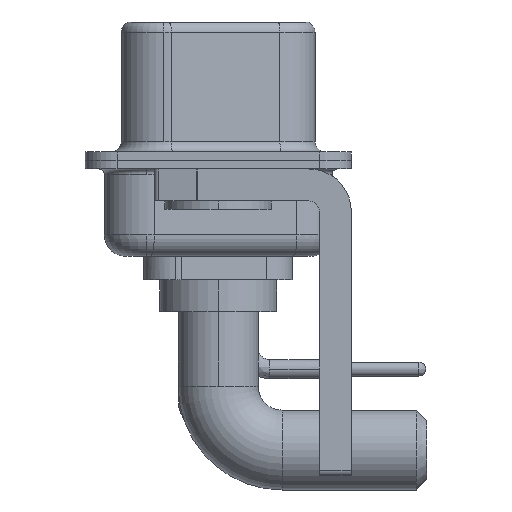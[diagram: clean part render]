
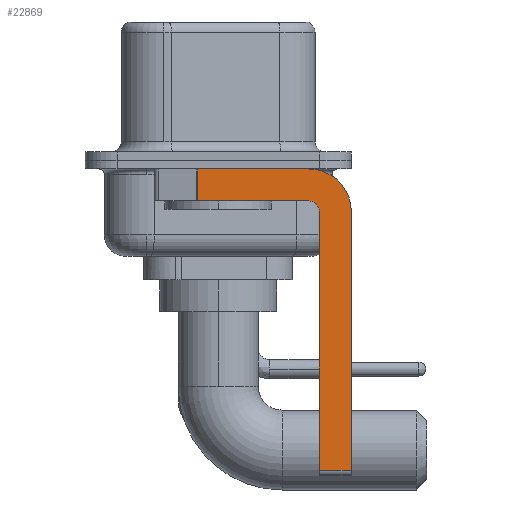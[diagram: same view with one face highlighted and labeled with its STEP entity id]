
A CAD part, left-side view. The second image highlights one B-rep face of the part: STEP entity #22869.
In plain terms, the highlighted planar face has unit normal (-1, 0, 0).
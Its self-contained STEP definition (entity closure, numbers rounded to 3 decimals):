
#163 = DIRECTION ( 'NONE',  ( 0., 0., -1. ) ) ;
#426 = DIRECTION ( 'NONE',  ( 0., -1., 0. ) ) ;
#742 = VERTEX_POINT ( 'NONE', #19148 ) ;
#838 = LINE ( 'NONE', #15015, #1181 ) ;
#1181 = VECTOR ( 'NONE', #22207, 1000. ) ;
#1190 = DIRECTION ( 'NONE',  ( 0., 0., -1. ) ) ;
#1272 = ORIENTED_EDGE ( 'NONE', *, *, #23228, .F. ) ;
#1300 = CARTESIAN_POINT ( 'NONE',  ( -2.9, -6.25, -2.4 ) ) ;
#1931 = ORIENTED_EDGE ( 'NONE', *, *, #2383, .F. ) ;
#2244 = CARTESIAN_POINT ( 'NONE',  ( -2.9, -4.25, -0.4 ) ) ;
#2383 = EDGE_CURVE ( 'NONE', #20773, #4508, #5707, .T. ) ;
#2916 = LINE ( 'NONE', #20500, #12174 ) ;
#3069 = VERTEX_POINT ( 'NONE', #10581 ) ;
#3169 = EDGE_CURVE ( 'NONE', #21324, #742, #18062, .T. ) ;
#3731 = VERTEX_POINT ( 'NONE', #15408 ) ;
#3820 = ORIENTED_EDGE ( 'NONE', *, *, #17250, .F. ) ;
#4007 = DIRECTION ( 'NONE',  ( 0., -1., 0. ) ) ;
#4075 = EDGE_CURVE ( 'NONE', #4508, #5373, #6496, .T. ) ;
#4508 = VERTEX_POINT ( 'NONE', #2244 ) ;
#4547 = CARTESIAN_POINT ( 'NONE',  ( -2.9, 0.978, -1.9 ) ) ;
#4710 = LINE ( 'NONE', #17585, #20706 ) ;
#5373 = VERTEX_POINT ( 'NONE', #1300 ) ;
#5699 = VECTOR ( 'NONE', #426, 1000. ) ;
#5707 = LINE ( 'NONE', #12840, #5699 ) ;
#6210 = AXIS2_PLACEMENT_3D ( 'NONE', #18989, #6334, #20876 ) ;
#6334 = DIRECTION ( 'NONE',  ( 1., 0., 0. ) ) ;
#6496 = CIRCLE ( 'NONE', #22203, 2. ) ;
#6719 = EDGE_LOOP ( 'NONE', ( #1931, #12902, #19871, #18921, #1272, #19207, #3820, #21828 ) ) ;
#7537 = CARTESIAN_POINT ( 'NONE',  ( -2.9, -4.25, -14.55 ) ) ;
#8010 = EDGE_CURVE ( 'NONE', #3069, #3731, #23111, .T. ) ;
#8795 = LINE ( 'NONE', #18158, #18171 ) ;
#8961 = CARTESIAN_POINT ( 'NONE',  ( -2.9, -4.25, -2.4 ) ) ;
#9198 = DIRECTION ( 'NONE',  ( 1., 0., 0. ) ) ;
#9677 = DIRECTION ( 'NONE',  ( -1., 0., 0. ) ) ;
#10581 = CARTESIAN_POINT ( 'NONE',  ( -2.9, -4.75, -2.4 ) ) ;
#11459 = CARTESIAN_POINT ( 'NONE',  ( -2.9, 0.978, -0.4 ) ) ;
#12174 = VECTOR ( 'NONE', #15442, 1000. ) ;
#12453 = VECTOR ( 'NONE', #4007, 1000. ) ;
#12569 = AXIS2_PLACEMENT_3D ( 'NONE', #13302, #9677, #20108 ) ;
#12840 = CARTESIAN_POINT ( 'NONE',  ( -2.9, 3., -0.4 ) ) ;
#12902 = ORIENTED_EDGE ( 'NONE', *, *, #18894, .T. ) ;
#13053 = PLANE ( 'NONE',  #6210 ) ;
#13302 = CARTESIAN_POINT ( 'NONE',  ( -2.9, -4.25, -2.4 ) ) ;
#15015 = CARTESIAN_POINT ( 'NONE',  ( -2.9, -6.25, -2.4 ) ) ;
#15237 = FACE_OUTER_BOUND ( 'NONE', #6719, .T. ) ;
#15408 = CARTESIAN_POINT ( 'NONE',  ( -2.9, -4.25, -1.9 ) ) ;
#15442 = DIRECTION ( 'NONE',  ( 0., 0., 1. ) ) ;
#16509 = DIRECTION ( 'NONE',  ( 0., 1., 0. ) ) ;
#17250 = EDGE_CURVE ( 'NONE', #5373, #742, #838, .T. ) ;
#17585 = CARTESIAN_POINT ( 'NONE',  ( -2.9, 0.978, -1.9 ) ) ;
#17716 = CARTESIAN_POINT ( 'NONE',  ( -2.9, -4.75, -14.55 ) ) ;
#18062 = LINE ( 'NONE', #7537, #12453 ) ;
#18158 = CARTESIAN_POINT ( 'NONE',  ( -2.9, -4.25, -1.9 ) ) ;
#18171 = VECTOR ( 'NONE', #16509, 1000. ) ;
#18894 = EDGE_CURVE ( 'NONE', #20773, #20658, #4710, .T. ) ;
#18921 = ORIENTED_EDGE ( 'NONE', *, *, #8010, .F. ) ;
#18989 = CARTESIAN_POINT ( 'NONE',  ( -2.9, -4.25, -2.4 ) ) ;
#19148 = CARTESIAN_POINT ( 'NONE',  ( -2.9, -6.25, -14.55 ) ) ;
#19207 = ORIENTED_EDGE ( 'NONE', *, *, #3169, .T. ) ;
#19871 = ORIENTED_EDGE ( 'NONE', *, *, #23078, .F. ) ;
#20108 = DIRECTION ( 'NONE',  ( 0., 0., 1. ) ) ;
#20500 = CARTESIAN_POINT ( 'NONE',  ( -2.9, -4.75, -14.8 ) ) ;
#20658 = VERTEX_POINT ( 'NONE', #4547 ) ;
#20706 = VECTOR ( 'NONE', #1190, 1000. ) ;
#20773 = VERTEX_POINT ( 'NONE', #11459 ) ;
#20876 = DIRECTION ( 'NONE',  ( 0., 0., -1. ) ) ;
#21324 = VERTEX_POINT ( 'NONE', #17716 ) ;
#21828 = ORIENTED_EDGE ( 'NONE', *, *, #4075, .F. ) ;
#22203 = AXIS2_PLACEMENT_3D ( 'NONE', #8961, #9198, #163 ) ;
#22207 = DIRECTION ( 'NONE',  ( 0., 0., -1. ) ) ;
#22869 = ADVANCED_FACE ( 'NONE', ( #15237 ), #13053, .F. ) ;
#23078 = EDGE_CURVE ( 'NONE', #3731, #20658, #8795, .T. ) ;
#23111 = CIRCLE ( 'NONE', #12569, 0.5 ) ;
#23228 = EDGE_CURVE ( 'NONE', #21324, #3069, #2916, .T. ) ;
